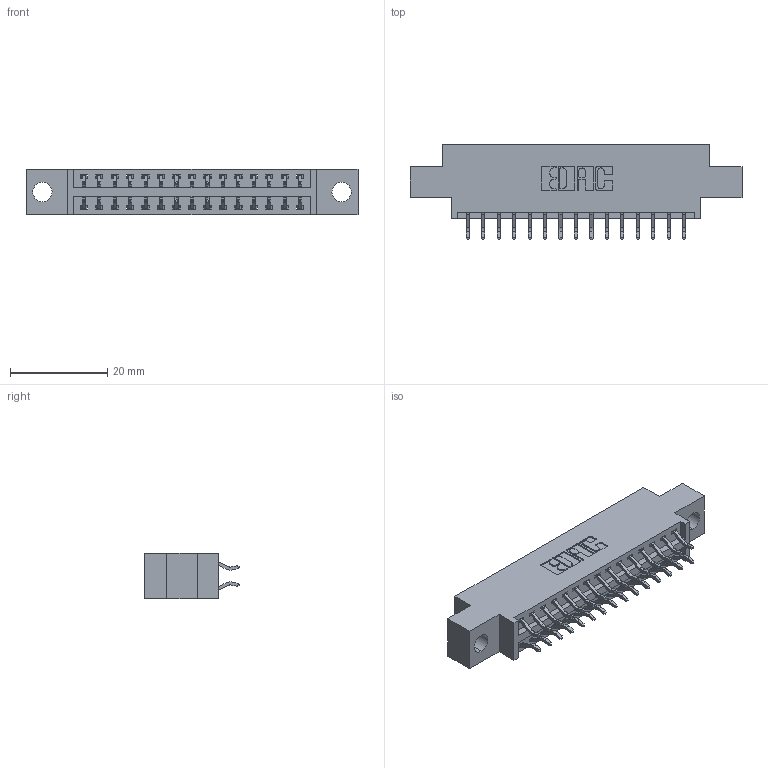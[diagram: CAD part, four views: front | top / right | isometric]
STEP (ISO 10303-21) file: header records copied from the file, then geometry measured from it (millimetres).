
FILE_DESCRIPTION (( 'STEP AP203' ), '1' );
FILE_NAME ('346-030-556-804.STEP', '2022-05-19T16:54:03', ( '' ), ( '' ), 'SwSTEP 2.0', 'SolidWorks 2020', '' );
FILE_SCHEMA (( 'CONFIG_CONTROL_DESIGN' ));
Length unit declared in the file: inch
Products named in the file (3): 346 Part_0.170 Offset - 0.156 Dia-TH; 345-292-001_556 Tail; 346-030-556-804
Assembly tree (31 placements, depth 2):
  346-030-556-804
    346 Part_0.170 Offset - 0.156 Dia-TH
    345-292-001_556 Tail  x30
Bounding box: 68.2 x 19.57 x 9.4 mm (x, y, z)
Volume: 6178.8 mm3; surface area: 8068.4 mm2
Topology: 31 solids, 31 shells, 1880 faces, 5567 edges, 3670 vertices
Faces by surface type: plane 1264, cylinder 616
Entity records: 14195 total; most frequent: CARTESIAN_POINT 2398, ORIENTED_EDGE 2318, DIRECTION 2151, EDGE_CURVE 1159, LINE 959, VECTOR 959, VERTEX_POINT 770, AXIS2_PLACEMENT_3D 596
